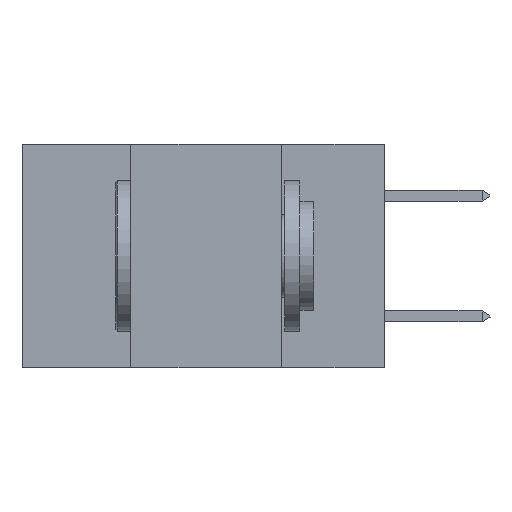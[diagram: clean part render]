
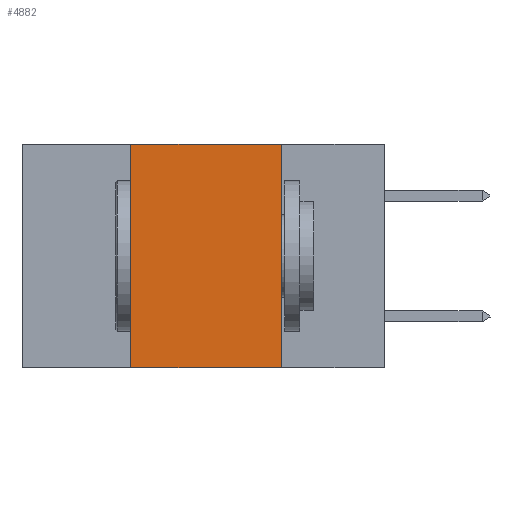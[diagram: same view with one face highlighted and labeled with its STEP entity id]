
A CAD part, left-side view. The second image highlights one B-rep face of the part: STEP entity #4882.
In plain terms, the highlighted planar face has unit normal (-1, 0, 0).
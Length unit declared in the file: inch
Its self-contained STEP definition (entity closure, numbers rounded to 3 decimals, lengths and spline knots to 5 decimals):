
#1136 = FACE_OUTER_BOUND ( 'NONE', #10222, .T. ) ;
#1633 = ORIENTED_EDGE ( 'NONE', *, *, #13810, .F. ) ;
#4882 = ADVANCED_FACE ( 'NONE', ( #1136 ), #24680, .F. ) ;
#5014 = VECTOR ( 'NONE', #6472, 39.37008 ) ;
#5925 = VECTOR ( 'NONE', #24308, 39.37008 ) ;
#6412 = CARTESIAN_POINT ( 'NONE',  ( 0., 0.42, -0.37 ) ) ;
#6472 = DIRECTION ( 'NONE',  ( 0., 0., -1. ) ) ;
#10222 = EDGE_LOOP ( 'NONE', ( #17806, #1633, #18474, #23953 ) ) ;
#10529 = CARTESIAN_POINT ( 'NONE',  ( 0., 0.6, 0. ) ) ;
#10778 = VERTEX_POINT ( 'NONE', #13329 ) ;
#11207 = EDGE_CURVE ( 'NONE', #25621, #10778, #19883, .T. ) ;
#11301 = EDGE_CURVE ( 'NONE', #22723, #15040, #11329, .T. ) ;
#11329 = LINE ( 'NONE', #18482, #5014 ) ;
#13329 = CARTESIAN_POINT ( 'NONE',  ( 0., 0.42, 0. ) ) ;
#13574 = VECTOR ( 'NONE', #16194, 39.37008 ) ;
#13810 = EDGE_CURVE ( 'NONE', #10778, #22723, #21139, .T. ) ;
#15040 = VERTEX_POINT ( 'NONE', #21230 ) ;
#16194 = DIRECTION ( 'NONE',  ( 0., 0., 1. ) ) ;
#17685 = DIRECTION ( 'NONE',  ( 1., 0., 0. ) ) ;
#17806 = ORIENTED_EDGE ( 'NONE', *, *, #11301, .F. ) ;
#18474 = ORIENTED_EDGE ( 'NONE', *, *, #11207, .F. ) ;
#18482 = CARTESIAN_POINT ( 'NONE',  ( 0., 0.17, 0. ) ) ;
#18893 = AXIS2_PLACEMENT_3D ( 'NONE', #10529, #17685, #20060 ) ;
#19121 = CARTESIAN_POINT ( 'NONE',  ( 0., 0.6, -0.37 ) ) ;
#19211 = DIRECTION ( 'NONE',  ( 0., -1., 0. ) ) ;
#19883 = LINE ( 'NONE', #30390, #13574 ) ;
#20060 = DIRECTION ( 'NONE',  ( 0., 0., -1. ) ) ;
#21139 = LINE ( 'NONE', #26509, #5925 ) ;
#21230 = CARTESIAN_POINT ( 'NONE',  ( 0., 0.17, -0.37 ) ) ;
#22723 = VERTEX_POINT ( 'NONE', #28972 ) ;
#23953 = ORIENTED_EDGE ( 'NONE', *, *, #25999, .T. ) ;
#24308 = DIRECTION ( 'NONE',  ( 0., -1., 0. ) ) ;
#24680 = PLANE ( 'NONE',  #18893 ) ;
#25621 = VERTEX_POINT ( 'NONE', #6412 ) ;
#25999 = EDGE_CURVE ( 'NONE', #25621, #15040, #29820, .T. ) ;
#26509 = CARTESIAN_POINT ( 'NONE',  ( 0., 0.6, 0. ) ) ;
#28972 = CARTESIAN_POINT ( 'NONE',  ( 0., 0.17, 0. ) ) ;
#29449 = VECTOR ( 'NONE', #19211, 39.37008 ) ;
#29820 = LINE ( 'NONE', #19121, #29449 ) ;
#30390 = CARTESIAN_POINT ( 'NONE',  ( 0., 0.42, 0. ) ) ;
